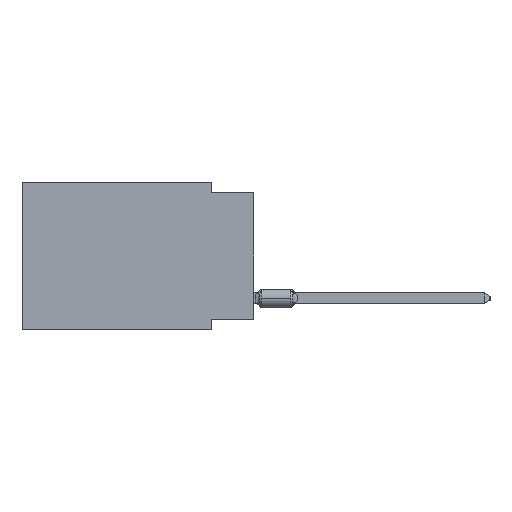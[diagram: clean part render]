
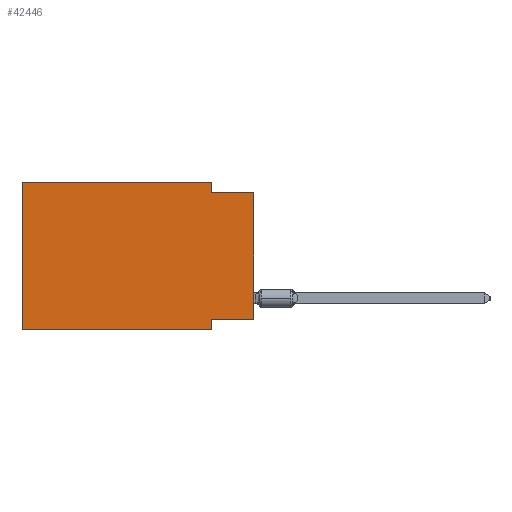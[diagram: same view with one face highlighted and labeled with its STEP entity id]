
A CAD part, left-side view. The second image highlights one B-rep face of the part: STEP entity #42446.
In plain terms, the highlighted planar face has unit normal (-1, 0, 0).
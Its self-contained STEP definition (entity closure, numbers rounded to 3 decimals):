
#693 = CARTESIAN_POINT ( 'NONE',  ( 0., 0., -0.635 ) ) ;
#1081 = LINE ( 'NONE', #25971, #69291 ) ;
#6584 = CARTESIAN_POINT ( 'NONE',  ( 0., 2.54, -8.255 ) ) ;
#8646 = VECTOR ( 'NONE', #54070, 1000. ) ;
#8945 = EDGE_CURVE ( 'NONE', #44904, #47242, #9366, .T. ) ;
#9366 = LINE ( 'NONE', #20954, #48421 ) ;
#13336 = EDGE_CURVE ( 'NONE', #34841, #44904, #26657, .T. ) ;
#15350 = EDGE_CURVE ( 'NONE', #34841, #21811, #44038, .T. ) ;
#15647 = DIRECTION ( 'NONE',  ( 0., 0., 1. ) ) ;
#15915 = EDGE_CURVE ( 'NONE', #66057, #47242, #30718, .T. ) ;
#16577 = EDGE_CURVE ( 'NONE', #64083, #21811, #18232, .T. ) ;
#17699 = CARTESIAN_POINT ( 'NONE',  ( 0., 2.54, 0. ) ) ;
#17921 = VECTOR ( 'NONE', #71842, 1000. ) ;
#18232 = LINE ( 'NONE', #693, #67087 ) ;
#18843 = CARTESIAN_POINT ( 'NONE',  ( 0., 0., -0.635 ) ) ;
#20954 = CARTESIAN_POINT ( 'NONE',  ( 0., 2.54, -8.89 ) ) ;
#21044 = EDGE_CURVE ( 'NONE', #32957, #64083, #47015, .T. ) ;
#21811 = VERTEX_POINT ( 'NONE', #18843 ) ;
#24382 = CARTESIAN_POINT ( 'NONE',  ( 0., 2.54, -8.89 ) ) ;
#24959 = ORIENTED_EDGE ( 'NONE', *, *, #53218, .F. ) ;
#25971 = CARTESIAN_POINT ( 'NONE',  ( 0., 13.97, 0. ) ) ;
#26657 = LINE ( 'NONE', #49060, #17921 ) ;
#30266 = ORIENTED_EDGE ( 'NONE', *, *, #8945, .F. ) ;
#30718 = LINE ( 'NONE', #48629, #37214 ) ;
#30822 = DIRECTION ( 'NONE',  ( 0., -1., 0. ) ) ;
#31300 = CARTESIAN_POINT ( 'NONE',  ( 0., 2.54, 0. ) ) ;
#32957 = VERTEX_POINT ( 'NONE', #17699 ) ;
#33000 = VERTEX_POINT ( 'NONE', #63613 ) ;
#34841 = VERTEX_POINT ( 'NONE', #73201 ) ;
#35923 = EDGE_LOOP ( 'NONE', ( #56825, #37690, #59486, #24959, #64671, #36250, #30266, #52519 ) ) ;
#36250 = ORIENTED_EDGE ( 'NONE', *, *, #15915, .T. ) ;
#37214 = VECTOR ( 'NONE', #53481, 1000. ) ;
#37690 = ORIENTED_EDGE ( 'NONE', *, *, #16577, .F. ) ;
#38436 = DIRECTION ( 'NONE',  ( 0., 0., -1. ) ) ;
#39643 = VECTOR ( 'NONE', #30822, 1000. ) ;
#42446 = ADVANCED_FACE ( 'NONE', ( #67557 ), #72429, .F. ) ;
#44038 = LINE ( 'NONE', #66809, #58641 ) ;
#44904 = VERTEX_POINT ( 'NONE', #6584 ) ;
#46253 = DIRECTION ( 'NONE',  ( 0., -1., 0. ) ) ;
#47015 = LINE ( 'NONE', #31300, #8646 ) ;
#47242 = VERTEX_POINT ( 'NONE', #24382 ) ;
#48421 = VECTOR ( 'NONE', #60901, 1000. ) ;
#48629 = CARTESIAN_POINT ( 'NONE',  ( 0., 13.97, -8.89 ) ) ;
#49060 = CARTESIAN_POINT ( 'NONE',  ( 0., 0., -8.255 ) ) ;
#49642 = CARTESIAN_POINT ( 'NONE',  ( 0., 13.97, 0. ) ) ;
#51745 = DIRECTION ( 'NONE',  ( 1., 0., 0. ) ) ;
#52519 = ORIENTED_EDGE ( 'NONE', *, *, #13336, .F. ) ;
#53218 = EDGE_CURVE ( 'NONE', #33000, #32957, #53580, .T. ) ;
#53481 = DIRECTION ( 'NONE',  ( 0., -1., 0. ) ) ;
#53580 = LINE ( 'NONE', #58461, #39643 ) ;
#53663 = CARTESIAN_POINT ( 'NONE',  ( 0., 2.54, -0.635 ) ) ;
#54070 = DIRECTION ( 'NONE',  ( 0., 0., -1. ) ) ;
#56825 = ORIENTED_EDGE ( 'NONE', *, *, #15350, .T. ) ;
#58461 = CARTESIAN_POINT ( 'NONE',  ( 0., 13.97, 0. ) ) ;
#58641 = VECTOR ( 'NONE', #15647, 1000. ) ;
#58893 = EDGE_CURVE ( 'NONE', #66057, #33000, #1081, .T. ) ;
#59486 = ORIENTED_EDGE ( 'NONE', *, *, #21044, .F. ) ;
#60901 = DIRECTION ( 'NONE',  ( 0., 0., -1. ) ) ;
#63381 = AXIS2_PLACEMENT_3D ( 'NONE', #49642, #51745, #38436 ) ;
#63613 = CARTESIAN_POINT ( 'NONE',  ( 0., 13.97, 0. ) ) ;
#64083 = VERTEX_POINT ( 'NONE', #53663 ) ;
#64671 = ORIENTED_EDGE ( 'NONE', *, *, #58893, .F. ) ;
#66057 = VERTEX_POINT ( 'NONE', #73437 ) ;
#66809 = CARTESIAN_POINT ( 'NONE',  ( 0., 0., 0. ) ) ;
#67087 = VECTOR ( 'NONE', #46253, 1000. ) ;
#67557 = FACE_OUTER_BOUND ( 'NONE', #35923, .T. ) ;
#69291 = VECTOR ( 'NONE', #71893, 1000. ) ;
#71842 = DIRECTION ( 'NONE',  ( 0., 1., 0. ) ) ;
#71893 = DIRECTION ( 'NONE',  ( 0., 0., 1. ) ) ;
#72429 = PLANE ( 'NONE',  #63381 ) ;
#73201 = CARTESIAN_POINT ( 'NONE',  ( 0., 0., -8.255 ) ) ;
#73437 = CARTESIAN_POINT ( 'NONE',  ( 0., 13.97, -8.89 ) ) ;
